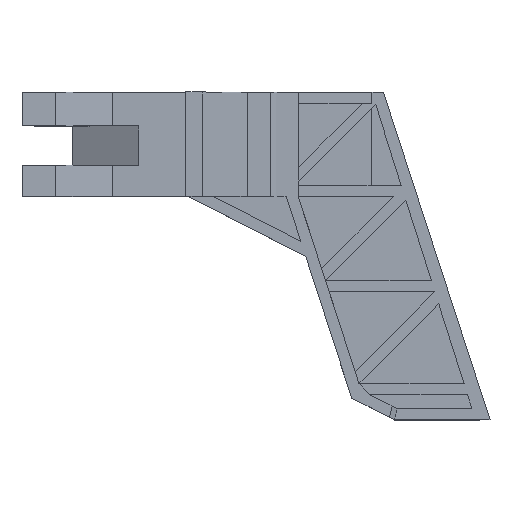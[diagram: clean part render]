
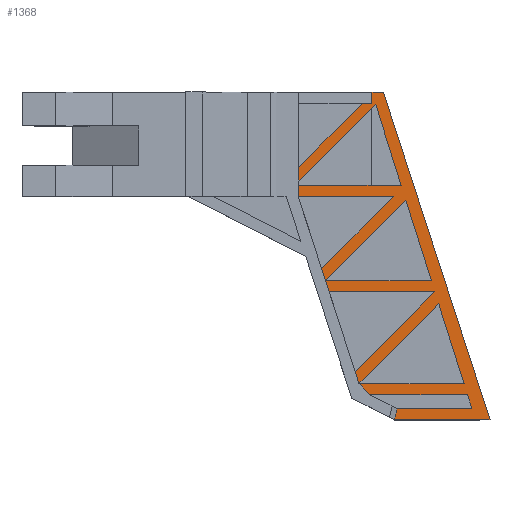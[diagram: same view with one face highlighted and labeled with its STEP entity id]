
A CAD part, top view. The second image highlights one B-rep face of the part: STEP entity #1368.
In plain terms, the highlighted planar face has unit normal (0, 0, 1).
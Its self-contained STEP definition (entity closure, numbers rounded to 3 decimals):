
#66=FACE_OUTER_BOUND('',#139,.T.);
#139=EDGE_LOOP('',(#1100,#1101,#1102,#1103,#1104,#1105,#1106,#1107,#1108,
#1109,#1110,#1111,#1112,#1113,#1114,#1115,#1116,#1117,#1118,#1119,#1120,
#1121,#1122,#1123,#1124,#1125,#1126,#1127,#1128,#1129,#1130));
#174=LINE('',#1838,#364);
#194=LINE('',#1880,#384);
#202=LINE('',#1896,#392);
#209=LINE('',#1910,#399);
#214=LINE('',#1921,#404);
#217=LINE('',#1926,#407);
#226=LINE('',#1942,#416);
#257=LINE('',#2006,#447);
#268=LINE('',#2028,#458);
#269=LINE('',#2029,#459);
#272=LINE('',#2037,#462);
#275=LINE('',#2043,#465);
#278=LINE('',#2047,#468);
#281=LINE('',#2054,#471);
#284=LINE('',#2060,#474);
#287=LINE('',#2064,#477);
#292=LINE('',#2075,#482);
#295=LINE('',#2081,#485);
#298=LINE('',#2085,#488);
#301=LINE('',#2093,#491);
#304=LINE('',#2099,#494);
#308=LINE('',#2106,#498);
#310=LINE('',#2108,#500);
#311=LINE('',#2110,#501);
#314=LINE('',#2116,#504);
#317=LINE('',#2120,#507);
#321=LINE('',#2129,#511);
#323=LINE('',#2132,#513);
#325=LINE('',#2137,#515);
#326=LINE('',#2139,#516);
#327=LINE('',#2140,#517);
#364=VECTOR('',#1494,10.);
#384=VECTOR('',#1520,10.);
#392=VECTOR('',#1534,10.);
#399=VECTOR('',#1545,10.);
#404=VECTOR('',#1552,10.);
#407=VECTOR('',#1557,10.);
#416=VECTOR('',#1570,10.);
#447=VECTOR('',#1617,10.);
#458=VECTOR('',#1632,10.);
#459=VECTOR('',#1633,10.);
#462=VECTOR('',#1638,10.);
#465=VECTOR('',#1643,10.);
#468=VECTOR('',#1648,10.);
#471=VECTOR('',#1653,10.);
#474=VECTOR('',#1658,10.);
#477=VECTOR('',#1663,10.);
#482=VECTOR('',#1672,10.);
#485=VECTOR('',#1677,10.);
#488=VECTOR('',#1682,10.);
#491=VECTOR('',#1687,10.);
#494=VECTOR('',#1692,10.);
#498=VECTOR('',#1698,10.);
#500=VECTOR('',#1700,10.);
#501=VECTOR('',#1701,10.);
#504=VECTOR('',#1706,10.);
#507=VECTOR('',#1711,10.);
#511=VECTOR('',#1721,10.);
#513=VECTOR('',#1725,10.);
#515=VECTOR('',#1731,10.);
#516=VECTOR('',#1732,10.);
#517=VECTOR('',#1733,10.);
#551=VERTEX_POINT('',#1831);
#554=VERTEX_POINT('',#1836);
#572=VERTEX_POINT('',#1878);
#573=VERTEX_POINT('',#1879);
#577=VERTEX_POINT('',#1894);
#578=VERTEX_POINT('',#1895);
#582=VERTEX_POINT('',#1907);
#583=VERTEX_POINT('',#1909);
#587=VERTEX_POINT('',#1918);
#588=VERTEX_POINT('',#1920);
#594=VERTEX_POINT('',#1940);
#618=VERTEX_POINT('',#2003);
#619=VERTEX_POINT('',#2005);
#628=VERTEX_POINT('',#2027);
#631=VERTEX_POINT('',#2034);
#632=VERTEX_POINT('',#2036);
#634=VERTEX_POINT('',#2042);
#637=VERTEX_POINT('',#2053);
#639=VERTEX_POINT('',#2059);
#643=VERTEX_POINT('',#2074);
#645=VERTEX_POINT('',#2080);
#648=VERTEX_POINT('',#2090);
#649=VERTEX_POINT('',#2092);
#651=VERTEX_POINT('',#2098);
#654=VERTEX_POINT('',#2109);
#656=VERTEX_POINT('',#2115);
#658=VERTEX_POINT('',#2128);
#659=VERTEX_POINT('',#2136);
#660=VERTEX_POINT('',#2138);
#679=EDGE_CURVE('',#551,#554,#174,.T.);
#699=EDGE_CURVE('',#572,#573,#194,.T.);
#707=EDGE_CURVE('',#577,#578,#202,.T.);
#714=EDGE_CURVE('',#583,#582,#209,.T.);
#719=EDGE_CURVE('',#588,#587,#214,.T.);
#722=EDGE_CURVE('',#582,#588,#217,.T.);
#731=EDGE_CURVE('',#587,#594,#226,.T.);
#763=EDGE_CURVE('',#619,#618,#257,.T.);
#775=EDGE_CURVE('',#628,#583,#268,.T.);
#776=EDGE_CURVE('',#618,#628,#269,.T.);
#779=EDGE_CURVE('',#632,#631,#272,.T.);
#782=EDGE_CURVE('',#634,#632,#275,.T.);
#785=EDGE_CURVE('',#631,#634,#278,.T.);
#788=EDGE_CURVE('',#637,#572,#281,.T.);
#791=EDGE_CURVE('',#639,#637,#284,.T.);
#794=EDGE_CURVE('',#572,#639,#287,.T.);
#799=EDGE_CURVE('',#643,#551,#292,.T.);
#802=EDGE_CURVE('',#645,#643,#295,.T.);
#805=EDGE_CURVE('',#573,#645,#298,.T.);
#808=EDGE_CURVE('',#649,#648,#301,.T.);
#811=EDGE_CURVE('',#651,#649,#304,.T.);
#815=EDGE_CURVE('',#648,#572,#308,.T.);
#817=EDGE_CURVE('',#631,#651,#310,.T.);
#818=EDGE_CURVE('',#654,#631,#311,.T.);
#821=EDGE_CURVE('',#656,#654,#314,.T.);
#824=EDGE_CURVE('',#578,#656,#317,.T.);
#828=EDGE_CURVE('',#658,#577,#321,.T.);
#830=EDGE_CURVE('',#594,#658,#323,.T.);
#832=EDGE_CURVE('',#554,#659,#325,.T.);
#833=EDGE_CURVE('',#659,#660,#326,.T.);
#834=EDGE_CURVE('',#660,#619,#327,.T.);
#1100=ORIENTED_EDGE('',*,*,#699,.T.);
#1101=ORIENTED_EDGE('',*,*,#805,.T.);
#1102=ORIENTED_EDGE('',*,*,#802,.T.);
#1103=ORIENTED_EDGE('',*,*,#799,.T.);
#1104=ORIENTED_EDGE('',*,*,#679,.T.);
#1105=ORIENTED_EDGE('',*,*,#832,.T.);
#1106=ORIENTED_EDGE('',*,*,#833,.T.);
#1107=ORIENTED_EDGE('',*,*,#834,.T.);
#1108=ORIENTED_EDGE('',*,*,#763,.T.);
#1109=ORIENTED_EDGE('',*,*,#776,.T.);
#1110=ORIENTED_EDGE('',*,*,#775,.T.);
#1111=ORIENTED_EDGE('',*,*,#714,.T.);
#1112=ORIENTED_EDGE('',*,*,#722,.T.);
#1113=ORIENTED_EDGE('',*,*,#719,.T.);
#1114=ORIENTED_EDGE('',*,*,#731,.T.);
#1115=ORIENTED_EDGE('',*,*,#830,.T.);
#1116=ORIENTED_EDGE('',*,*,#828,.T.);
#1117=ORIENTED_EDGE('',*,*,#707,.T.);
#1118=ORIENTED_EDGE('',*,*,#824,.T.);
#1119=ORIENTED_EDGE('',*,*,#821,.T.);
#1120=ORIENTED_EDGE('',*,*,#818,.T.);
#1121=ORIENTED_EDGE('',*,*,#785,.T.);
#1122=ORIENTED_EDGE('',*,*,#782,.T.);
#1123=ORIENTED_EDGE('',*,*,#779,.T.);
#1124=ORIENTED_EDGE('',*,*,#817,.T.);
#1125=ORIENTED_EDGE('',*,*,#811,.T.);
#1126=ORIENTED_EDGE('',*,*,#808,.T.);
#1127=ORIENTED_EDGE('',*,*,#815,.T.);
#1128=ORIENTED_EDGE('',*,*,#794,.T.);
#1129=ORIENTED_EDGE('',*,*,#791,.T.);
#1130=ORIENTED_EDGE('',*,*,#788,.T.);
#1299=PLANE('',#1455);
#1368=ADVANCED_FACE('',(#66),#1299,.T.);
#1455=AXIS2_PLACEMENT_3D('',#2135,#1729,#1730);
#1494=DIRECTION('',(-0.234,-0.972,0.));
#1520=DIRECTION('',(0.7,-0.714,0.));
#1534=DIRECTION('',(-0.039,-0.999,0.));
#1545=DIRECTION('',(-0.707,-0.707,0.));
#1552=DIRECTION('',(0.707,0.707,0.));
#1557=DIRECTION('',(0.,-1.,0.));
#1570=DIRECTION('',(0.309,-0.951,0.));
#1617=DIRECTION('',(-1.,0.,0.));
#1632=DIRECTION('',(-1.,0.,0.));
#1633=DIRECTION('',(0.,-1.,0.));
#1638=DIRECTION('',(-1.,0.,0.));
#1643=DIRECTION('',(0.302,-0.953,0.));
#1648=DIRECTION('',(0.707,0.707,0.));
#1653=DIRECTION('',(-1.,0.,0.));
#1658=DIRECTION('',(0.302,-0.953,0.));
#1663=DIRECTION('',(0.707,0.707,0.));
#1672=DIRECTION('',(-1.,-0.003,0.));
#1677=DIRECTION('',(0.302,-0.953,0.));
#1682=DIRECTION('',(1.,0.,0.));
#1687=DIRECTION('',(-0.707,-0.707,0.));
#1692=DIRECTION('',(1.,0.,0.));
#1698=DIRECTION('',(0.309,-0.951,0.));
#1700=DIRECTION('',(0.309,-0.951,0.));
#1701=DIRECTION('',(0.309,-0.951,0.));
#1706=DIRECTION('',(-0.707,-0.707,0.));
#1711=DIRECTION('',(1.,0.,0.));
#1721=DIRECTION('',(-1.,0.,0.));
#1725=DIRECTION('',(0.302,-0.953,0.));
#1729=DIRECTION('center_axis',(0.,0.,1.));
#1730=DIRECTION('ref_axis',(1.,0.,0.));
#1731=DIRECTION('',(1.,0.,0.));
#1732=DIRECTION('',(1.,0.003,0.));
#1733=DIRECTION('',(-0.309,0.951,0.));
#1831=CARTESIAN_POINT('',(29.236,-19.793,-1.5));
#1836=CARTESIAN_POINT('',(28.995,-20.793,-1.5));
#1838=CARTESIAN_POINT('',(30.514,-14.486,-1.5));
#1878=CARTESIAN_POINT('',(25.85,-17.586,-1.5));
#1879=CARTESIAN_POINT('',(26.785,-18.54,-1.5));
#1880=CARTESIAN_POINT('',(23.063,-14.743,-1.5));
#1894=CARTESIAN_POINT('',(20.5,0.,-1.5));
#1895=CARTESIAN_POINT('',(20.461,-1.,-1.5));
#1896=CARTESIAN_POINT('',(20.362,-3.561,-1.5));
#1907=CARTESIAN_POINT('',(20.5,1.589,-1.5));
#1909=CARTESIAN_POINT('',(26.161,7.25,-1.5));
#1910=CARTESIAN_POINT('',(20.5,1.589,-1.5));
#1918=CARTESIAN_POINT('',(27.323,7.165,-1.5));
#1920=CARTESIAN_POINT('',(20.5,0.342,-1.5));
#1921=CARTESIAN_POINT('',(20.5,0.342,-1.5));
#1926=CARTESIAN_POINT('',(20.5,-3.136,-1.5));
#1940=CARTESIAN_POINT('',(27.396,6.941,-1.5));
#1942=CARTESIAN_POINT('',(27.396,6.941,-1.5));
#2003=CARTESIAN_POINT('',(27.,8.25,-1.5));
#2005=CARTESIAN_POINT('',(28.022,8.25,-1.5));
#2006=CARTESIAN_POINT('',(28.103,8.25,-1.5));
#2027=CARTESIAN_POINT('',(27.,7.25,-1.5));
#2028=CARTESIAN_POINT('',(19.5,7.25,-1.5));
#2029=CARTESIAN_POINT('',(27.,8.25,-1.5));
#2034=CARTESIAN_POINT('',(22.879,-8.443,-1.5));
#2036=CARTESIAN_POINT('',(32.263,-8.443,-1.5));
#2037=CARTESIAN_POINT('',(22.879,-8.443,-1.5));
#2042=CARTESIAN_POINT('',(30.008,-1.315,-1.5));
#2043=CARTESIAN_POINT('',(27.396,6.941,-1.5));
#2047=CARTESIAN_POINT('',(29.615,-1.707,-1.5));
#2053=CARTESIAN_POINT('',(35.156,-17.586,-1.5));
#2054=CARTESIAN_POINT('',(25.85,-17.586,-1.5));
#2059=CARTESIAN_POINT('',(32.92,-10.517,-1.5));
#2060=CARTESIAN_POINT('',(27.396,6.941,-1.5));
#2064=CARTESIAN_POINT('',(32.92,-10.517,-1.5));
#2074=CARTESIAN_POINT('',(35.848,-19.772,-1.5));
#2075=CARTESIAN_POINT('',(29.236,-19.793,-1.5));
#2080=CARTESIAN_POINT('',(35.458,-18.54,-1.5));
#2081=CARTESIAN_POINT('',(27.396,6.941,-1.5));
#2085=CARTESIAN_POINT('',(35.458,-18.54,-1.5));
#2090=CARTESIAN_POINT('',(25.504,-16.519,-1.5));
#2092=CARTESIAN_POINT('',(32.58,-9.443,-1.5));
#2093=CARTESIAN_POINT('',(32.58,-9.443,-1.5));
#2098=CARTESIAN_POINT('',(23.204,-9.443,-1.5));
#2099=CARTESIAN_POINT('',(23.204,-9.443,-1.5));
#2106=CARTESIAN_POINT('',(24.104,-12.213,-1.5));
#2108=CARTESIAN_POINT('',(24.104,-12.213,-1.5));
#2109=CARTESIAN_POINT('',(22.533,-7.376,-1.5));
#2110=CARTESIAN_POINT('',(24.104,-12.213,-1.5));
#2115=CARTESIAN_POINT('',(28.908,-1.,-1.5));
#2116=CARTESIAN_POINT('',(28.908,-1.,-1.5));
#2120=CARTESIAN_POINT('',(28.908,-1.,-1.5));
#2128=CARTESIAN_POINT('',(29.592,0.,-1.5));
#2129=CARTESIAN_POINT('',(19.5,0.,-1.5));
#2132=CARTESIAN_POINT('',(27.396,6.941,-1.5));
#2135=CARTESIAN_POINT('Origin',(24.108,-6.271,-1.5));
#2136=CARTESIAN_POINT('',(36.355,-20.793,-1.5));
#2137=CARTESIAN_POINT('',(28.995,-20.793,-1.5));
#2138=CARTESIAN_POINT('',(37.457,-20.789,-1.5));
#2139=CARTESIAN_POINT('',(36.355,-20.793,-1.5));
#2140=CARTESIAN_POINT('',(37.457,-20.789,-1.5));
